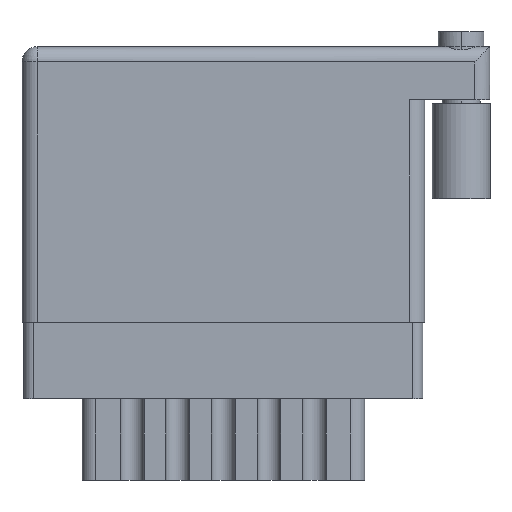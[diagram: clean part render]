
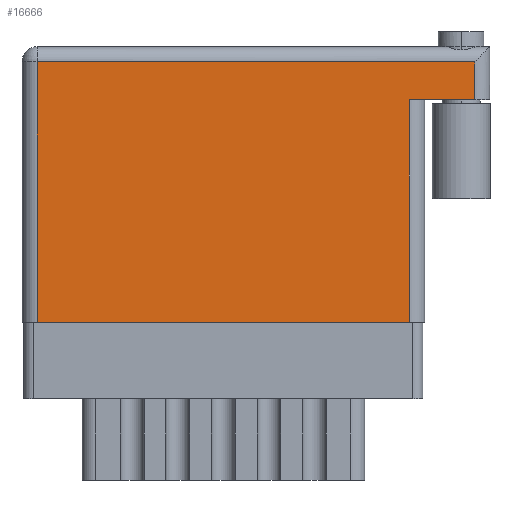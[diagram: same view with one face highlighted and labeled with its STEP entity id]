
A CAD part, front view. The second image highlights one B-rep face of the part: STEP entity #16666.
In plain terms, the highlighted face is planar.
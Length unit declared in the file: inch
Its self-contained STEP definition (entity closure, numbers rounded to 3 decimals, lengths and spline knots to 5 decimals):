
#152 = PLANE ( 'NONE',  #14403 ) ;
#352 = EDGE_CURVE ( 'NONE', #10748, #381, #1921, .T. ) ;
#381 = VERTEX_POINT ( 'NONE', #13943 ) ;
#977 = CARTESIAN_POINT ( 'NONE',  ( 0.05, 0., 0. ) ) ;
#1867 = VECTOR ( 'NONE', #23011, 39.37008 ) ;
#1921 = LINE ( 'NONE', #21672, #20288 ) ;
#2512 = VECTOR ( 'NONE', #23147, 39.37008 ) ;
#3412 = LINE ( 'NONE', #11515, #2512 ) ;
#5098 = CARTESIAN_POINT ( 'NONE',  ( 0., 0.856, 0. ) ) ;
#5496 = DIRECTION ( 'NONE',  ( 0., -1., 0. ) ) ;
#5556 = CARTESIAN_POINT ( 'NONE',  ( 1.489, 0.731, 0. ) ) ;
#6672 = VECTOR ( 'NONE', #5496, 39.37008 ) ;
#7410 = ORIENTED_EDGE ( 'NONE', *, *, #352, .T. ) ;
#9058 = EDGE_CURVE ( 'NONE', #15601, #12112, #12944, .T. ) ;
#9887 = DIRECTION ( 'NONE',  ( 1., 0., 0. ) ) ;
#10348 = DIRECTION ( 'NONE',  ( 0., 0., -1. ) ) ;
#10732 = LINE ( 'NONE', #20419, #19428 ) ;
#10748 = VERTEX_POINT ( 'NONE', #977 ) ;
#11284 = VECTOR ( 'NONE', #20154, 39.37008 ) ;
#11515 = CARTESIAN_POINT ( 'NONE',  ( 1.275, 0.731, 0. ) ) ;
#11987 = ORIENTED_EDGE ( 'NONE', *, *, #23858, .T. ) ;
#12112 = VERTEX_POINT ( 'NONE', #21916 ) ;
#12944 = LINE ( 'NONE', #5098, #1867 ) ;
#13943 = CARTESIAN_POINT ( 'NONE',  ( 1.275, 0., 0. ) ) ;
#14395 = ORIENTED_EDGE ( 'NONE', *, *, #16797, .F. ) ;
#14403 = AXIS2_PLACEMENT_3D ( 'NONE', #23824, #10348, #21858 ) ;
#15141 = VERTEX_POINT ( 'NONE', #16465 ) ;
#15441 = LINE ( 'NONE', #23411, #6672 ) ;
#15601 = VERTEX_POINT ( 'NONE', #22566 ) ;
#16465 = CARTESIAN_POINT ( 'NONE',  ( 1.275, 0.731, 0. ) ) ;
#16666 = ADVANCED_FACE ( 'NONE', ( #19907 ), #152, .F. ) ;
#16797 = EDGE_CURVE ( 'NONE', #24759, #15141, #10732, .T. ) ;
#17132 = ORIENTED_EDGE ( 'NONE', *, *, #23978, .T. ) ;
#18723 = DIRECTION ( 'NONE',  ( -1., 0., 0. ) ) ;
#19428 = VECTOR ( 'NONE', #18723, 39.37008 ) ;
#19907 = FACE_OUTER_BOUND ( 'NONE', #24955, .T. ) ;
#19909 = LINE ( 'NONE', #22127, #11284 ) ;
#20154 = DIRECTION ( 'NONE',  ( 0., 1., 0. ) ) ;
#20288 = VECTOR ( 'NONE', #9887, 39.37008 ) ;
#20419 = CARTESIAN_POINT ( 'NONE',  ( 1.539, 0.731, 0. ) ) ;
#21672 = CARTESIAN_POINT ( 'NONE',  ( 0., 0., 0. ) ) ;
#21858 = DIRECTION ( 'NONE',  ( -1., 0., 0. ) ) ;
#21916 = CARTESIAN_POINT ( 'NONE',  ( 0.05, 0.856, 0. ) ) ;
#22127 = CARTESIAN_POINT ( 'NONE',  ( 1.489, 0.906, 0. ) ) ;
#22566 = CARTESIAN_POINT ( 'NONE',  ( 1.489, 0.856, 0. ) ) ;
#22722 = ORIENTED_EDGE ( 'NONE', *, *, #23689, .T. ) ;
#23011 = DIRECTION ( 'NONE',  ( -1., 0., 0. ) ) ;
#23147 = DIRECTION ( 'NONE',  ( 0., 1., 0. ) ) ;
#23411 = CARTESIAN_POINT ( 'NONE',  ( 0.05, 0., 0. ) ) ;
#23689 = EDGE_CURVE ( 'NONE', #24759, #15601, #19909, .T. ) ;
#23824 = CARTESIAN_POINT ( 'NONE',  ( 0., 0.906, 0. ) ) ;
#23858 = EDGE_CURVE ( 'NONE', #381, #15141, #3412, .T. ) ;
#23978 = EDGE_CURVE ( 'NONE', #12112, #10748, #15441, .T. ) ;
#24759 = VERTEX_POINT ( 'NONE', #5556 ) ;
#24955 = EDGE_LOOP ( 'NONE', ( #7410, #11987, #14395, #22722, #25566, #17132 ) ) ;
#25566 = ORIENTED_EDGE ( 'NONE', *, *, #9058, .T. ) ;
